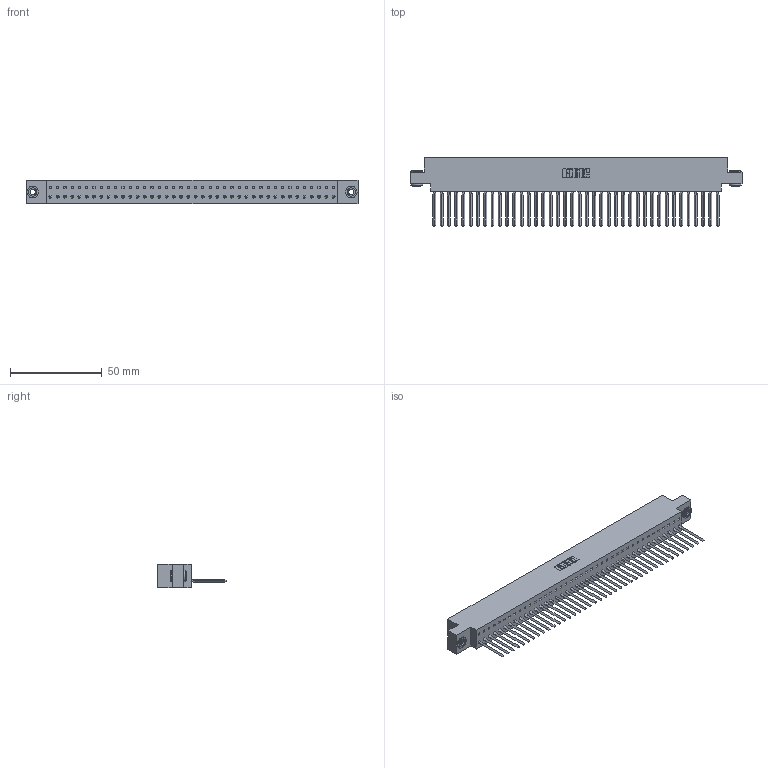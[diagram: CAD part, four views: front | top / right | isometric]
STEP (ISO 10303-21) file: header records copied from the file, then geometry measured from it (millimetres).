
FILE_DESCRIPTION (( 'STEP AP203' ), '1' );
FILE_NAME ('317-040-541-603.STEP', '2020-02-28T00:19:32', ( '' ), ( '' ), 'SwSTEP 2.0', 'SolidWorks 2016', '' );
FILE_SCHEMA (( 'CONFIG_CONTROL_DESIGN' ));
Length unit declared in the file: inch
Products named in the file (4): 345-250-002_345-250-002-102; 317-040-541-603; 317 Part_.156 Dia - TH; 317-290-002_541
Assembly tree (43 placements, depth 2):
  317-040-541-603
    317 Part_.156 Dia - TH
    317-290-002_541  x40
    345-250-002_345-250-002-102  x2
Bounding box: 181.2 x 37.34 x 12.7 mm (x, y, z)
Volume: 29343 mm3; surface area: 41611.7 mm2
Topology: 43 solids, 43 shells, 6220 faces, 17711 edges, 11510 vertices
Faces by surface type: plane 5028, cylinder 1024, bspline 160, cone 8
Entity records: 59017 total; most frequent: CARTESIAN_POINT 11100, ORIENTED_EDGE 10386, DIRECTION 8571, EDGE_CURVE 5193, LINE 4805, VECTOR 4805, VERTEX_POINT 3452, AXIS2_PLACEMENT_3D 1883
